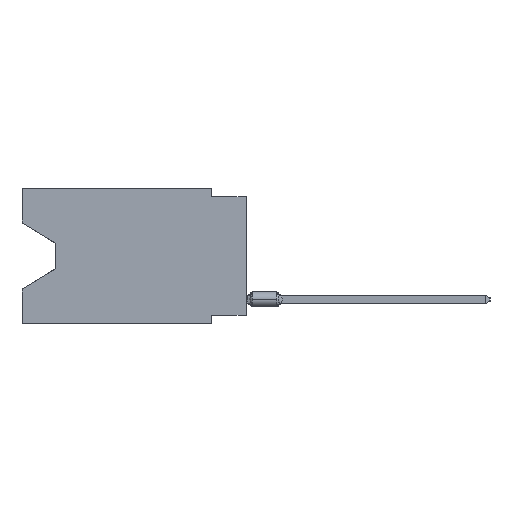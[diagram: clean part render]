
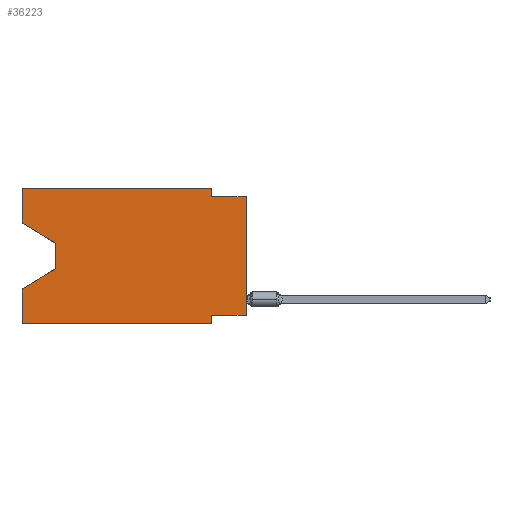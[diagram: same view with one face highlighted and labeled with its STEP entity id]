
A CAD part, left-side view. The second image highlights one B-rep face of the part: STEP entity #36223.
In plain terms, the highlighted planar face has unit normal (-1, 0, 0).
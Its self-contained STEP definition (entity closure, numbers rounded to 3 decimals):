
#471 = ORIENTED_EDGE ( 'NONE', *, *, #59586, .T. ) ;
#1050 = PLANE ( 'NONE',  #58164 ) ;
#1574 = ORIENTED_EDGE ( 'NONE', *, *, #9053, .T. ) ;
#1714 = VERTEX_POINT ( 'NONE', #42681 ) ;
#1804 = VECTOR ( 'NONE', #6719, 1000. ) ;
#1829 = EDGE_CURVE ( 'NONE', #9288, #24995, #25177, .T. ) ;
#2338 = DIRECTION ( 'NONE',  ( 0., 0., 1. ) ) ;
#2569 = VERTEX_POINT ( 'NONE', #10900 ) ;
#4797 = VERTEX_POINT ( 'NONE', #43758 ) ;
#6063 = DIRECTION ( 'NONE',  ( 0., -1., 0. ) ) ;
#6160 = DIRECTION ( 'NONE',  ( 0., -1., 0. ) ) ;
#6719 = DIRECTION ( 'NONE',  ( 0., 0., -1. ) ) ;
#6759 = LINE ( 'NONE', #20301, #31220 ) ;
#8124 = ORIENTED_EDGE ( 'NONE', *, *, #58125, .F. ) ;
#8927 = LINE ( 'NONE', #22472, #49214 ) ;
#9053 = EDGE_CURVE ( 'NONE', #24995, #11959, #43355, .T. ) ;
#9159 = CARTESIAN_POINT ( 'NONE',  ( 0., 2.54, 0. ) ) ;
#9288 = VERTEX_POINT ( 'NONE', #27263 ) ;
#10462 = DIRECTION ( 'NONE',  ( 0., 0., -1. ) ) ;
#10888 = ORIENTED_EDGE ( 'NONE', *, *, #1829, .T. ) ;
#10900 = CARTESIAN_POINT ( 'NONE',  ( 0., 16.383, -9.906 ) ) ;
#11069 = LINE ( 'NONE', #21189, #18600 ) ;
#11150 = CARTESIAN_POINT ( 'NONE',  ( 0., 0., -0.635 ) ) ;
#11959 = VERTEX_POINT ( 'NONE', #32100 ) ;
#12485 = ORIENTED_EDGE ( 'NONE', *, *, #31843, .F. ) ;
#12733 = EDGE_LOOP ( 'NONE', ( #54102, #10888, #1574, #8124, #471, #12485, #35225, #26883, #23656, #14361, #16698, #20387 ) ) ;
#13255 = DIRECTION ( 'NONE',  ( 0., -1., 0. ) ) ;
#14361 = ORIENTED_EDGE ( 'NONE', *, *, #55189, .F. ) ;
#14663 = CARTESIAN_POINT ( 'NONE',  ( 0., 16.383, 0. ) ) ;
#16698 = ORIENTED_EDGE ( 'NONE', *, *, #56341, .F. ) ;
#18386 = CARTESIAN_POINT ( 'NONE',  ( 0., 0., -9.271 ) ) ;
#18600 = VECTOR ( 'NONE', #6160, 1000. ) ;
#19061 = VECTOR ( 'NONE', #6063, 1000. ) ;
#19672 = CARTESIAN_POINT ( 'NONE',  ( 0., 2.54, -9.906 ) ) ;
#20301 = CARTESIAN_POINT ( 'NONE',  ( 0., 16.383, -2.546 ) ) ;
#20387 = ORIENTED_EDGE ( 'NONE', *, *, #59643, .F. ) ;
#20579 = LINE ( 'NONE', #39318, #41269 ) ;
#20847 = CARTESIAN_POINT ( 'NONE',  ( 0., 16.383, -2.546 ) ) ;
#21189 = CARTESIAN_POINT ( 'NONE',  ( 0., 0., -0.635 ) ) ;
#22472 = CARTESIAN_POINT ( 'NONE',  ( 0., 16.383, 0. ) ) ;
#23067 = EDGE_CURVE ( 'NONE', #4797, #52424, #23316, .T. ) ;
#23316 = LINE ( 'NONE', #18386, #33948 ) ;
#23330 = CARTESIAN_POINT ( 'NONE',  ( 0., 16.383, 0. ) ) ;
#23624 = DIRECTION ( 'NONE',  ( 0., 1., 0. ) ) ;
#23656 = ORIENTED_EDGE ( 'NONE', *, *, #44438, .F. ) ;
#24995 = VERTEX_POINT ( 'NONE', #47950 ) ;
#25038 = EDGE_CURVE ( 'NONE', #34255, #9288, #6759, .T. ) ;
#25177 = LINE ( 'NONE', #43893, #1804 ) ;
#26299 = LINE ( 'NONE', #45025, #52406 ) ;
#26883 = ORIENTED_EDGE ( 'NONE', *, *, #36433, .T. ) ;
#27263 = CARTESIAN_POINT ( 'NONE',  ( 0., 13.97, -4.013 ) ) ;
#28921 = VECTOR ( 'NONE', #42664, 1000. ) ;
#29226 = DIRECTION ( 'NONE',  ( 0., 0., -1. ) ) ;
#29421 = LINE ( 'NONE', #53358, #19061 ) ;
#29846 = DIRECTION ( 'NONE',  ( 0., 0.855, -0.519 ) ) ;
#30748 = VERTEX_POINT ( 'NONE', #11150 ) ;
#31220 = VECTOR ( 'NONE', #58362, 1000. ) ;
#31843 = EDGE_CURVE ( 'NONE', #52424, #1714, #35223, .T. ) ;
#32100 = CARTESIAN_POINT ( 'NONE',  ( 0., 16.383, -7.36 ) ) ;
#32996 = DIRECTION ( 'NONE',  ( 1., 0., 0. ) ) ;
#33948 = VECTOR ( 'NONE', #23624, 1000. ) ;
#34255 = VERTEX_POINT ( 'NONE', #20847 ) ;
#35223 = LINE ( 'NONE', #19672, #51275 ) ;
#35225 = ORIENTED_EDGE ( 'NONE', *, *, #23067, .F. ) ;
#36223 = ADVANCED_FACE ( 'NONE', ( #47452 ), #1050, .F. ) ;
#36433 = EDGE_CURVE ( 'NONE', #4797, #30748, #36912, .T. ) ;
#36912 = LINE ( 'NONE', #55352, #56233 ) ;
#37906 = CARTESIAN_POINT ( 'NONE',  ( 0., 16.383, 0. ) ) ;
#39318 = CARTESIAN_POINT ( 'NONE',  ( 0., 2.54, 0. ) ) ;
#40981 = CARTESIAN_POINT ( 'NONE',  ( 0., 2.54, -9.271 ) ) ;
#41269 = VECTOR ( 'NONE', #29226, 1000. ) ;
#42664 = DIRECTION ( 'NONE',  ( 0., 0., 1. ) ) ;
#42681 = CARTESIAN_POINT ( 'NONE',  ( 0., 2.54, -9.906 ) ) ;
#43133 = DIRECTION ( 'NONE',  ( 0., 0., -1. ) ) ;
#43355 = LINE ( 'NONE', #57781, #56499 ) ;
#43758 = CARTESIAN_POINT ( 'NONE',  ( 0., 0., -9.271 ) ) ;
#43893 = CARTESIAN_POINT ( 'NONE',  ( 0., 13.97, -4.013 ) ) ;
#44438 = EDGE_CURVE ( 'NONE', #45472, #30748, #11069, .T. ) ;
#45025 = CARTESIAN_POINT ( 'NONE',  ( 0., 16.383, 0. ) ) ;
#45472 = VERTEX_POINT ( 'NONE', #47337 ) ;
#47337 = CARTESIAN_POINT ( 'NONE',  ( 0., 2.54, -0.635 ) ) ;
#47452 = FACE_OUTER_BOUND ( 'NONE', #12733, .T. ) ;
#47950 = CARTESIAN_POINT ( 'NONE',  ( 0., 13.97, -5.893 ) ) ;
#49214 = VECTOR ( 'NONE', #13255, 1000. ) ;
#51275 = VECTOR ( 'NONE', #10462, 1000. ) ;
#51589 = VERTEX_POINT ( 'NONE', #9159 ) ;
#52406 = VECTOR ( 'NONE', #2338, 1000. ) ;
#52424 = VERTEX_POINT ( 'NONE', #40981 ) ;
#53358 = CARTESIAN_POINT ( 'NONE',  ( 0., 16.383, -9.906 ) ) ;
#54102 = ORIENTED_EDGE ( 'NONE', *, *, #25038, .T. ) ;
#55189 = EDGE_CURVE ( 'NONE', #51589, #45472, #20579, .T. ) ;
#55352 = CARTESIAN_POINT ( 'NONE',  ( 0., 0., 0. ) ) ;
#56190 = LINE ( 'NONE', #23330, #28921 ) ;
#56233 = VECTOR ( 'NONE', #59657, 1000. ) ;
#56341 = EDGE_CURVE ( 'NONE', #59425, #51589, #8927, .T. ) ;
#56499 = VECTOR ( 'NONE', #29846, 1000. ) ;
#57781 = CARTESIAN_POINT ( 'NONE',  ( 0., 13.97, -5.893 ) ) ;
#58125 = EDGE_CURVE ( 'NONE', #2569, #11959, #56190, .T. ) ;
#58164 = AXIS2_PLACEMENT_3D ( 'NONE', #37906, #32996, #43133 ) ;
#58362 = DIRECTION ( 'NONE',  ( 0., -0.855, -0.519 ) ) ;
#59425 = VERTEX_POINT ( 'NONE', #14663 ) ;
#59586 = EDGE_CURVE ( 'NONE', #2569, #1714, #29421, .T. ) ;
#59643 = EDGE_CURVE ( 'NONE', #34255, #59425, #26299, .T. ) ;
#59657 = DIRECTION ( 'NONE',  ( 0., 0., 1. ) ) ;
